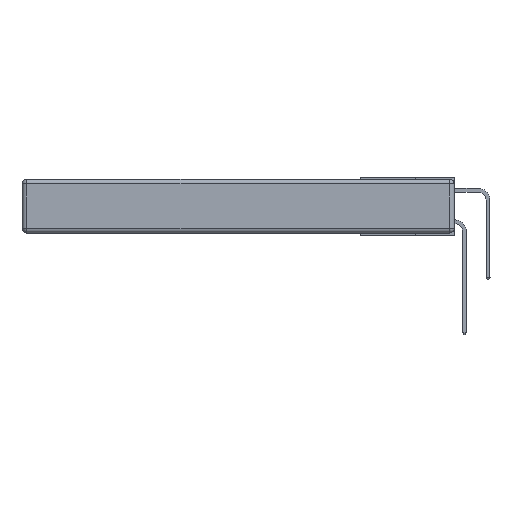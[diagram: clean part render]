
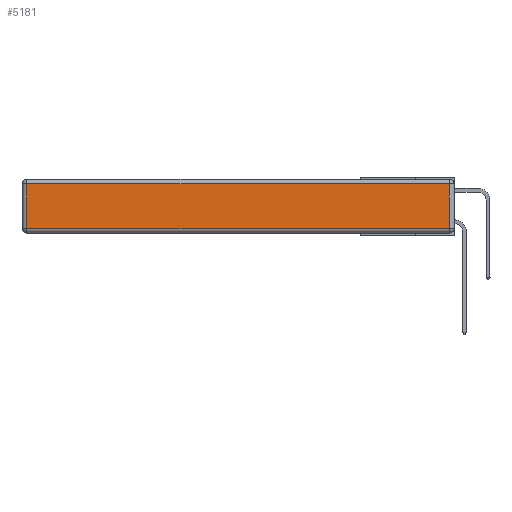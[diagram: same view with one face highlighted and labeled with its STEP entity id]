
A CAD part, left-side view. The second image highlights one B-rep face of the part: STEP entity #5181.
In plain terms, the highlighted planar face has unit normal (-1, 0, 0).
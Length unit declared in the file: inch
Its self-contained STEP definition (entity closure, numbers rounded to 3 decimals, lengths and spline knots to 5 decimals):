
#1401 = LINE ( 'NONE', #17024, #16570 ) ;
#2346 = EDGE_CURVE ( 'NONE', #13705, #4593, #16087, .T. ) ;
#2975 = CARTESIAN_POINT ( 'NONE',  ( 0., 0., -0.313 ) ) ;
#3379 = CARTESIAN_POINT ( 'NONE',  ( 0., 0.03, -0.03 ) ) ;
#3699 = VECTOR ( 'NONE', #11702, 39.37008 ) ;
#4593 = VERTEX_POINT ( 'NONE', #13079 ) ;
#5181 = ADVANCED_FACE ( 'NONE', ( #13920 ), #17959, .T. ) ;
#5480 = ORIENTED_EDGE ( 'NONE', *, *, #11604, .T. ) ;
#5739 = DIRECTION ( 'NONE',  ( 0., 0., -1. ) ) ;
#6086 = CARTESIAN_POINT ( 'NONE',  ( 0., 0., -0.343 ) ) ;
#6533 = ORIENTED_EDGE ( 'NONE', *, *, #16152, .T. ) ;
#7146 = CARTESIAN_POINT ( 'NONE',  ( 0., 2.72, -0.343 ) ) ;
#7481 = ORIENTED_EDGE ( 'NONE', *, *, #2346, .T. ) ;
#7690 = EDGE_LOOP ( 'NONE', ( #5480, #6533, #17905, #7481 ) ) ;
#10082 = DIRECTION ( 'NONE',  ( 0., -1., 0. ) ) ;
#10197 = CARTESIAN_POINT ( 'NONE',  ( 0., 2.72, -0.03 ) ) ;
#10719 = VERTEX_POINT ( 'NONE', #13504 ) ;
#11604 = EDGE_CURVE ( 'NONE', #4593, #10719, #15761, .T. ) ;
#11702 = DIRECTION ( 'NONE',  ( 0., 1., 0. ) ) ;
#12332 = VECTOR ( 'NONE', #10082, 39.37008 ) ;
#12640 = LINE ( 'NONE', #17745, #3699 ) ;
#13079 = CARTESIAN_POINT ( 'NONE',  ( 0., 2.72, -0.313 ) ) ;
#13312 = AXIS2_PLACEMENT_3D ( 'NONE', #6086, #14923, #13523 ) ;
#13412 = VERTEX_POINT ( 'NONE', #3379 ) ;
#13504 = CARTESIAN_POINT ( 'NONE',  ( 0., 0.03, -0.313 ) ) ;
#13523 = DIRECTION ( 'NONE',  ( 0., 0., 1. ) ) ;
#13705 = VERTEX_POINT ( 'NONE', #10197 ) ;
#13920 = FACE_OUTER_BOUND ( 'NONE', #7690, .T. ) ;
#14222 = VECTOR ( 'NONE', #5739, 39.37008 ) ;
#14923 = DIRECTION ( 'NONE',  ( -1., 0., 0. ) ) ;
#15761 = LINE ( 'NONE', #2975, #12332 ) ;
#16087 = LINE ( 'NONE', #7146, #14222 ) ;
#16152 = EDGE_CURVE ( 'NONE', #10719, #13412, #1401, .T. ) ;
#16348 = EDGE_CURVE ( 'NONE', #13412, #13705, #12640, .T. ) ;
#16570 = VECTOR ( 'NONE', #18300, 39.37008 ) ;
#17024 = CARTESIAN_POINT ( 'NONE',  ( 0., 0.03, -0.343 ) ) ;
#17745 = CARTESIAN_POINT ( 'NONE',  ( 0., 2.75, -0.03 ) ) ;
#17905 = ORIENTED_EDGE ( 'NONE', *, *, #16348, .T. ) ;
#17959 = PLANE ( 'NONE',  #13312 ) ;
#18300 = DIRECTION ( 'NONE',  ( 0., 0., 1. ) ) ;
